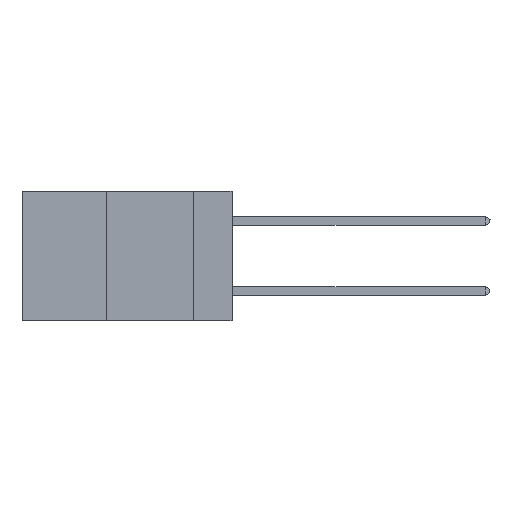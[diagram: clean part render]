
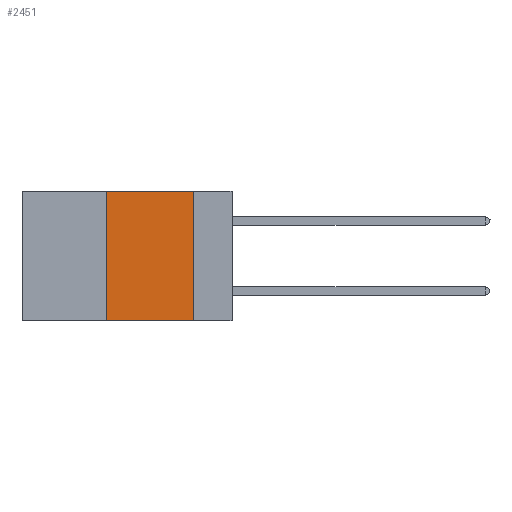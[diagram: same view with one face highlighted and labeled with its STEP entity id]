
A CAD part, left-side view. The second image highlights one B-rep face of the part: STEP entity #2451.
In plain terms, the highlighted planar face has unit normal (-1, 0, 0).
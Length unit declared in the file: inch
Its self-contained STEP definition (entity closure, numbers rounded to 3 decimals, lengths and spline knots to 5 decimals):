
#1079 = LINE ( 'NONE', #13979, #17710 ) ;
#2130 = PLANE ( 'NONE',  #16837 ) ;
#2451 = ADVANCED_FACE ( 'NONE', ( #4883 ), #2130, .F. ) ;
#4013 = CARTESIAN_POINT ( 'NONE',  ( 0., 0.36, 0. ) ) ;
#4173 = EDGE_LOOP ( 'NONE', ( #6058, #16079, #31553, #18588 ) ) ;
#4883 = FACE_OUTER_BOUND ( 'NONE', #4173, .T. ) ;
#6058 = ORIENTED_EDGE ( 'NONE', *, *, #26704, .F. ) ;
#6102 = EDGE_CURVE ( 'NONE', #37515, #12151, #10669, .T. ) ;
#6677 = DIRECTION ( 'NONE',  ( 0., 0., 1. ) ) ;
#10162 = VECTOR ( 'NONE', #33317, 39.37008 ) ;
#10600 = DIRECTION ( 'NONE',  ( 0., -1., 0. ) ) ;
#10669 = LINE ( 'NONE', #17625, #10162 ) ;
#10919 = VERTEX_POINT ( 'NONE', #15530 ) ;
#11741 = CARTESIAN_POINT ( 'NONE',  ( 0., 0.36, -0.37 ) ) ;
#12151 = VERTEX_POINT ( 'NONE', #37585 ) ;
#13221 = CARTESIAN_POINT ( 'NONE',  ( 0., 0.36, 0. ) ) ;
#13979 = CARTESIAN_POINT ( 'NONE',  ( 0., 0.6, 0. ) ) ;
#14056 = VECTOR ( 'NONE', #6677, 39.37008 ) ;
#14595 = DIRECTION ( 'NONE',  ( 1., 0., 0. ) ) ;
#15530 = CARTESIAN_POINT ( 'NONE',  ( 0., 0.11, 0. ) ) ;
#16079 = ORIENTED_EDGE ( 'NONE', *, *, #27945, .F. ) ;
#16837 = AXIS2_PLACEMENT_3D ( 'NONE', #41066, #14595, #27516 ) ;
#17625 = CARTESIAN_POINT ( 'NONE',  ( 0., 0.6, -0.37 ) ) ;
#17710 = VECTOR ( 'NONE', #10600, 39.37008 ) ;
#17714 = DIRECTION ( 'NONE',  ( 0., 0., -1. ) ) ;
#18588 = ORIENTED_EDGE ( 'NONE', *, *, #6102, .T. ) ;
#18740 = EDGE_CURVE ( 'NONE', #37515, #25531, #29521, .T. ) ;
#25531 = VERTEX_POINT ( 'NONE', #4013 ) ;
#26704 = EDGE_CURVE ( 'NONE', #10919, #12151, #37418, .T. ) ;
#27516 = DIRECTION ( 'NONE',  ( 0., 0., -1. ) ) ;
#27945 = EDGE_CURVE ( 'NONE', #25531, #10919, #1079, .T. ) ;
#29521 = LINE ( 'NONE', #13221, #14056 ) ;
#31553 = ORIENTED_EDGE ( 'NONE', *, *, #18740, .F. ) ;
#33317 = DIRECTION ( 'NONE',  ( 0., -1., 0. ) ) ;
#35311 = VECTOR ( 'NONE', #17714, 39.37008 ) ;
#37418 = LINE ( 'NONE', #40187, #35311 ) ;
#37515 = VERTEX_POINT ( 'NONE', #11741 ) ;
#37585 = CARTESIAN_POINT ( 'NONE',  ( 0., 0.11, -0.37 ) ) ;
#40187 = CARTESIAN_POINT ( 'NONE',  ( 0., 0.11, 0. ) ) ;
#41066 = CARTESIAN_POINT ( 'NONE',  ( 0., 0.6, 0. ) ) ;
